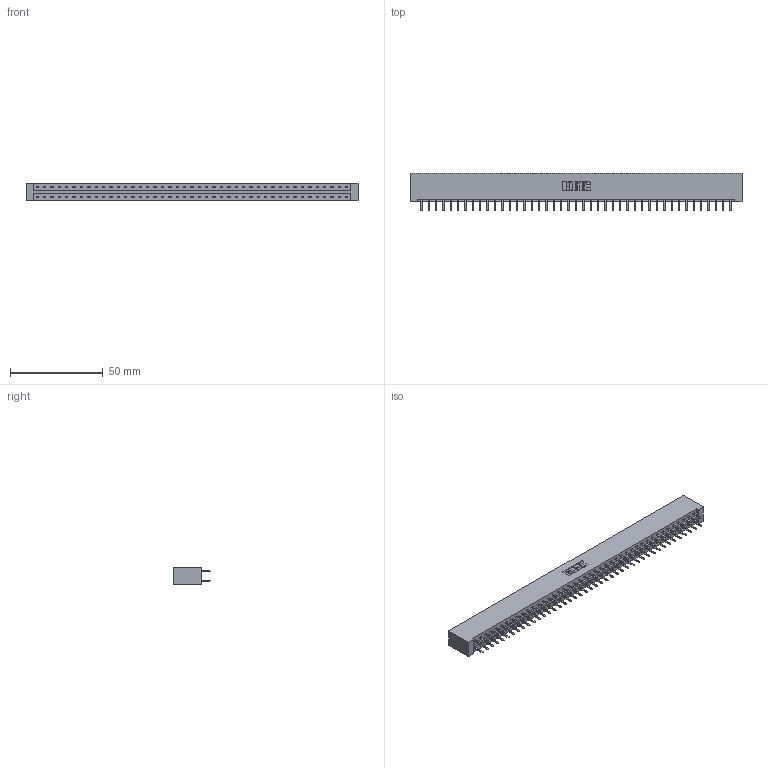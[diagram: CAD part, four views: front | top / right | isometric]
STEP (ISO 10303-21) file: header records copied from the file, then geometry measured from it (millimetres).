
FILE_DESCRIPTION (( 'STEP AP203' ), '1' );
FILE_NAME ('833-086-520-201.STEP', '2020-06-06T02:43:23', ( '' ), ( '' ), 'SwSTEP 2.0', 'SolidWorks 2020', '' );
FILE_SCHEMA (( 'CONFIG_CONTROL_DESIGN' ));
Length unit declared in the file: inch
Products named in the file (3): 833 Part_Lugless; 345-292-001_345-293-120; 833-086-520-201
Assembly tree (87 placements, depth 2):
  833-086-520-201
    833 Part_Lugless
    345-292-001_345-293-120  x86
Bounding box: 178.64 x 20.02 x 9.4 mm (x, y, z)
Volume: 18841.7 mm3; surface area: 22210.6 mm2
Topology: 87 solids, 87 shells, 4922 faces, 14305 edges, 9306 vertices
Faces by surface type: plane 3334, cylinder 1588
Entity records: 27371 total; most frequent: CARTESIAN_POINT 4546, ORIENTED_EDGE 4470, DIRECTION 3863, EDGE_CURVE 2235, VECTOR 2111, LINE 2111, VERTEX_POINT 1486, AXIS2_PLACEMENT_3D 876
